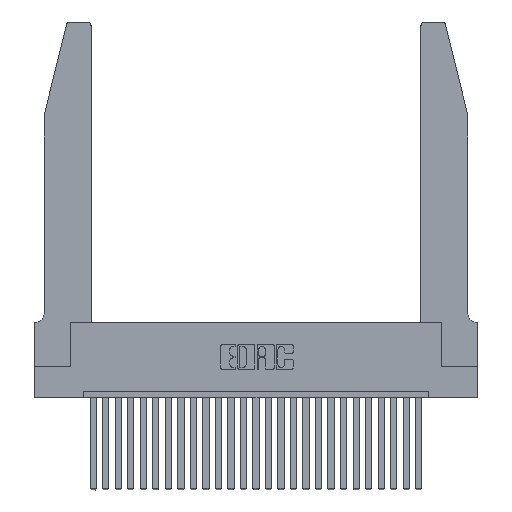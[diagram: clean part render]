
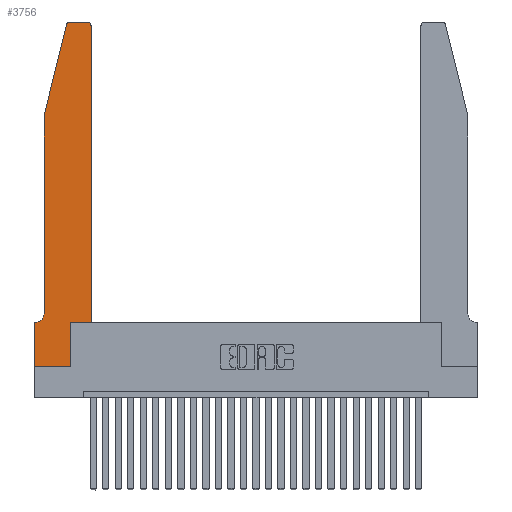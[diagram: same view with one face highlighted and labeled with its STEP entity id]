
A CAD part, top view. The second image highlights one B-rep face of the part: STEP entity #3756.
In plain terms, the highlighted planar face has unit normal (0, 0, 1).
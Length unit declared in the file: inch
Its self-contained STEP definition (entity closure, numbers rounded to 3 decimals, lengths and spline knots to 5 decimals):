
#148 = EDGE_CURVE ( 'NONE', #3166, #12750, #23459, .T. ) ;
#375 = VERTEX_POINT ( 'NONE', #15410 ) ;
#396 = CARTESIAN_POINT ( 'NONE',  ( 0.25487, 2.72718, 0.37 ) ) ;
#700 = DIRECTION ( 'NONE',  ( 1., 0., 0. ) ) ;
#955 = DIRECTION ( 'NONE',  ( -1., 0., 0. ) ) ;
#1287 = AXIS2_PLACEMENT_3D ( 'NONE', #9676, #14143, #22265 ) ;
#1606 = ORIENTED_EDGE ( 'NONE', *, *, #18622, .T. ) ;
#1755 = LINE ( 'NONE', #11282, #8905 ) ;
#2423 = CARTESIAN_POINT ( 'NONE',  ( 0.0755, 0.42, 0.37 ) ) ;
#2890 = CARTESIAN_POINT ( 'NONE',  ( 0.0055, 0.42, 0.37 ) ) ;
#3157 = LINE ( 'NONE', #21898, #15191 ) ;
#3166 = VERTEX_POINT ( 'NONE', #18965 ) ;
#3756 = ADVANCED_FACE ( 'NONE', ( #13312 ), #22091, .T. ) ;
#3864 = CARTESIAN_POINT ( 'NONE',  ( 0.0055, 0.35, 0.37 ) ) ;
#5145 = AXIS2_PLACEMENT_3D ( 'NONE', #7006, #7092, #15478 ) ;
#5542 = CARTESIAN_POINT ( 'NONE',  ( 0.0755, 2., 0.37 ) ) ;
#6242 = AXIS2_PLACEMENT_3D ( 'NONE', #7315, #11850, #24323 ) ;
#6796 = CARTESIAN_POINT ( 'NONE',  ( 0., 0., 0.37 ) ) ;
#6981 = VERTEX_POINT ( 'NONE', #24759 ) ;
#7006 = CARTESIAN_POINT ( 'NONE',  ( 0.284, 2.72, 0.37 ) ) ;
#7092 = DIRECTION ( 'NONE',  ( 0., 0., 1. ) ) ;
#7106 = LINE ( 'NONE', #24445, #17530 ) ;
#7315 = CARTESIAN_POINT ( 'NONE',  ( 0.4205, 2.72, 0.37 ) ) ;
#7321 = VECTOR ( 'NONE', #8901, 39.37008 ) ;
#7433 = ORIENTED_EDGE ( 'NONE', *, *, #21359, .T. ) ;
#7587 = VERTEX_POINT ( 'NONE', #7753 ) ;
#7739 = DIRECTION ( 'NONE',  ( 0., -1., 0. ) ) ;
#7753 = CARTESIAN_POINT ( 'NONE',  ( 0., 0., 0.37 ) ) ;
#7956 = DIRECTION ( 'NONE',  ( -0.239, -0.971, 0. ) ) ;
#8008 = LINE ( 'NONE', #6796, #20982 ) ;
#8279 = CARTESIAN_POINT ( 'NONE',  ( 0.0755, 0.35, 0.37 ) ) ;
#8402 = ORIENTED_EDGE ( 'NONE', *, *, #18279, .T. ) ;
#8775 = CARTESIAN_POINT ( 'NONE',  ( 0.2865, 0.35, 0.37 ) ) ;
#8872 = DIRECTION ( 'NONE',  ( 1., 0., 0. ) ) ;
#8901 = DIRECTION ( 'NONE',  ( 0., -1., 0. ) ) ;
#8905 = VECTOR ( 'NONE', #17275, 39.37008 ) ;
#9002 = CARTESIAN_POINT ( 'NONE',  ( 0.4505, 0.35, 0.37 ) ) ;
#9141 = VECTOR ( 'NONE', #7739, 39.37008 ) ;
#9584 = VECTOR ( 'NONE', #13354, 39.37008 ) ;
#9619 = VERTEX_POINT ( 'NONE', #2423 ) ;
#9626 = VERTEX_POINT ( 'NONE', #8775 ) ;
#9676 = CARTESIAN_POINT ( 'NONE',  ( 0., 0.35, 0.37 ) ) ;
#10112 = ORIENTED_EDGE ( 'NONE', *, *, #17445, .T. ) ;
#10405 = CIRCLE ( 'NONE', #26057, 0.07 ) ;
#11282 = CARTESIAN_POINT ( 'NONE',  ( 0.4505, 0.35, 0.37 ) ) ;
#11430 = ORIENTED_EDGE ( 'NONE', *, *, #23983, .T. ) ;
#11514 = ORIENTED_EDGE ( 'NONE', *, *, #24341, .T. ) ;
#11850 = DIRECTION ( 'NONE',  ( 0., 0., 1. ) ) ;
#11969 = EDGE_CURVE ( 'NONE', #13147, #9626, #14174, .T. ) ;
#12523 = VERTEX_POINT ( 'NONE', #13522 ) ;
#12750 = VERTEX_POINT ( 'NONE', #12752 ) ;
#12752 = CARTESIAN_POINT ( 'NONE',  ( 0.4205, 2.75, 0.37 ) ) ;
#13147 = VERTEX_POINT ( 'NONE', #13375 ) ;
#13312 = FACE_OUTER_BOUND ( 'NONE', #16990, .T. ) ;
#13354 = DIRECTION ( 'NONE',  ( 0., 1., 0. ) ) ;
#13375 = CARTESIAN_POINT ( 'NONE',  ( 0.2865, 0., 0.37 ) ) ;
#13522 = CARTESIAN_POINT ( 'NONE',  ( 0., 0.35, 0.37 ) ) ;
#14143 = DIRECTION ( 'NONE',  ( 0., 0., 1. ) ) ;
#14174 = LINE ( 'NONE', #23469, #9584 ) ;
#14367 = EDGE_CURVE ( 'NONE', #14567, #9619, #25328, .T. ) ;
#14567 = VERTEX_POINT ( 'NONE', #25967 ) ;
#14826 = CARTESIAN_POINT ( 'NONE',  ( 0., 0., 0.37 ) ) ;
#14907 = EDGE_CURVE ( 'NONE', #9619, #22919, #10405, .T. ) ;
#15191 = VECTOR ( 'NONE', #21712, 39.37008 ) ;
#15387 = VECTOR ( 'NONE', #700, 39.37008 ) ;
#15410 = CARTESIAN_POINT ( 'NONE',  ( 0.4505, 0.35, 0.37 ) ) ;
#15478 = DIRECTION ( 'NONE',  ( 1., 0., 0. ) ) ;
#15666 = ORIENTED_EDGE ( 'NONE', *, *, #148, .T. ) ;
#16212 = EDGE_CURVE ( 'NONE', #12750, #6981, #3157, .T. ) ;
#16924 = DIRECTION ( 'NONE',  ( -1., 0., 0. ) ) ;
#16990 = EDGE_LOOP ( 'NONE', ( #23447, #11430, #7433, #22107, #18040, #8402, #23253, #11514, #22897, #1606, #10112, #15666 ) ) ;
#17275 = DIRECTION ( 'NONE',  ( 0., 1., 0. ) ) ;
#17445 = EDGE_CURVE ( 'NONE', #375, #3166, #1755, .T. ) ;
#17530 = VECTOR ( 'NONE', #7956, 39.37008 ) ;
#18040 = ORIENTED_EDGE ( 'NONE', *, *, #14907, .T. ) ;
#18279 = EDGE_CURVE ( 'NONE', #22919, #12523, #22792, .T. ) ;
#18621 = VECTOR ( 'NONE', #16924, 39.37008 ) ;
#18622 = EDGE_CURVE ( 'NONE', #9626, #375, #24070, .T. ) ;
#18965 = CARTESIAN_POINT ( 'NONE',  ( 0.4505, 2.72, 0.37 ) ) ;
#19788 = DIRECTION ( 'NONE',  ( 0., 0., -1. ) ) ;
#20603 = VERTEX_POINT ( 'NONE', #396 ) ;
#20982 = VECTOR ( 'NONE', #8872, 39.37008 ) ;
#21359 = EDGE_CURVE ( 'NONE', #20603, #14567, #7106, .T. ) ;
#21712 = DIRECTION ( 'NONE',  ( -1., 0., 0. ) ) ;
#21898 = CARTESIAN_POINT ( 'NONE',  ( 0.2605, 2.75, 0.37 ) ) ;
#22091 = PLANE ( 'NONE',  #1287 ) ;
#22107 = ORIENTED_EDGE ( 'NONE', *, *, #14367, .T. ) ;
#22265 = DIRECTION ( 'NONE',  ( 1., 0., 0. ) ) ;
#22792 = LINE ( 'NONE', #8279, #18621 ) ;
#22897 = ORIENTED_EDGE ( 'NONE', *, *, #11969, .T. ) ;
#22919 = VERTEX_POINT ( 'NONE', #3864 ) ;
#23253 = ORIENTED_EDGE ( 'NONE', *, *, #25583, .T. ) ;
#23447 = ORIENTED_EDGE ( 'NONE', *, *, #16212, .T. ) ;
#23459 = CIRCLE ( 'NONE', #6242, 0.03 ) ;
#23469 = CARTESIAN_POINT ( 'NONE',  ( 0.2865, 0.35, 0.37 ) ) ;
#23983 = EDGE_CURVE ( 'NONE', #6981, #20603, #26831, .T. ) ;
#24070 = LINE ( 'NONE', #9002, #15387 ) ;
#24323 = DIRECTION ( 'NONE',  ( 1., 0., 0. ) ) ;
#24341 = EDGE_CURVE ( 'NONE', #7587, #13147, #8008, .T. ) ;
#24445 = CARTESIAN_POINT ( 'NONE',  ( 0.0755, 2., 0.37 ) ) ;
#24759 = CARTESIAN_POINT ( 'NONE',  ( 0.284, 2.75, 0.37 ) ) ;
#25127 = LINE ( 'NONE', #14826, #7321 ) ;
#25328 = LINE ( 'NONE', #5542, #9141 ) ;
#25583 = EDGE_CURVE ( 'NONE', #12523, #7587, #25127, .T. ) ;
#25967 = CARTESIAN_POINT ( 'NONE',  ( 0.0755, 2., 0.37 ) ) ;
#26057 = AXIS2_PLACEMENT_3D ( 'NONE', #2890, #19788, #955 ) ;
#26831 = CIRCLE ( 'NONE', #5145, 0.03 ) ;
